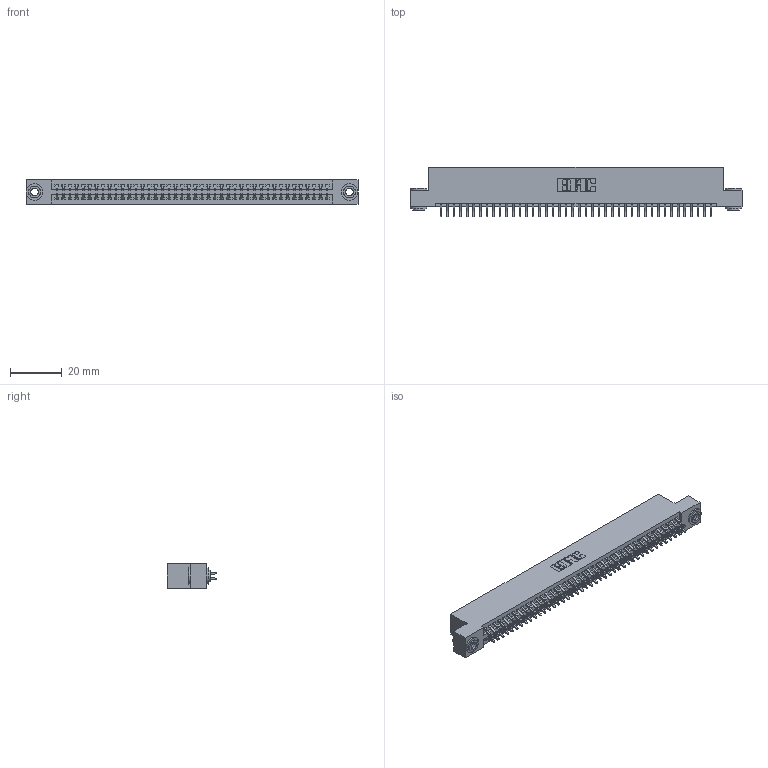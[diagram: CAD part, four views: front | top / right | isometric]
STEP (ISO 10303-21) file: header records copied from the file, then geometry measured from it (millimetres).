
FILE_DESCRIPTION (( 'STEP AP203' ), '1' );
FILE_NAME ('395-084-556-203.STEP', '2019-10-25T10:11:55', ( '' ), ( '' ), 'SwSTEP 2.0', 'SolidWorks 2016', '' );
FILE_SCHEMA (( 'CONFIG_CONTROL_DESIGN' ));
Length unit declared in the file: inch
Products named in the file (4): 395-084-556-203; 345 Part_Flush Mounting Lugs - 0.156 Dia-TH; 345-292-001_556 Tail; 345-250-002_345-250-002-102
Assembly tree (87 placements, depth 2):
  395-084-556-203
    345 Part_Flush Mounting Lugs - 0.156 Dia-TH
    345-292-001_556 Tail  x84
    345-250-002_345-250-002-102  x2
Bounding box: 127.89 x 19.24 x 9.4 mm (x, y, z)
Volume: 12439.3 mm3; surface area: 18518.8 mm2
Topology: 87 solids, 87 shells, 4868 faces, 14445 edges, 9514 vertices
Faces by surface type: plane 3198, cylinder 1662, cone 8
Entity records: 33824 total; most frequent: CARTESIAN_POINT 5659, ORIENTED_EDGE 5574, DIRECTION 5009, EDGE_CURVE 2787, LINE 2455, VECTOR 2455, VERTEX_POINT 1854, AXIS2_PLACEMENT_3D 1277
